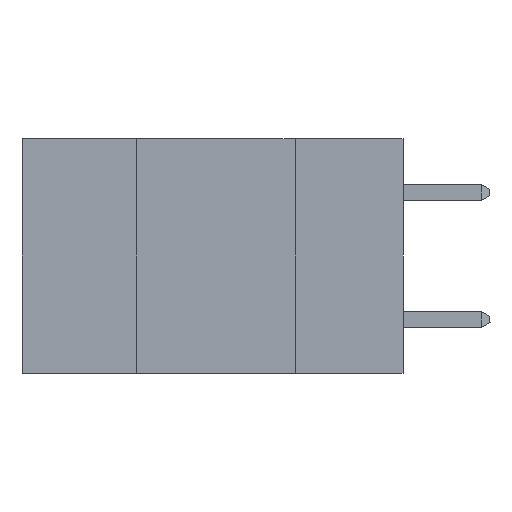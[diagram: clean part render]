
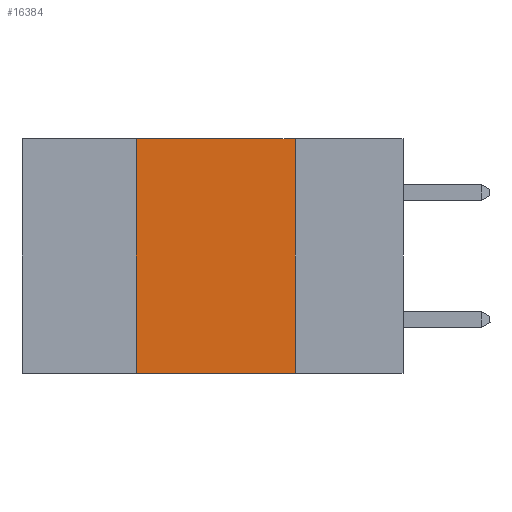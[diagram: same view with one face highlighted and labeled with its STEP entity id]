
A CAD part, left-side view. The second image highlights one B-rep face of the part: STEP entity #16384.
In plain terms, the highlighted planar face has unit normal (-1, 0, 0).
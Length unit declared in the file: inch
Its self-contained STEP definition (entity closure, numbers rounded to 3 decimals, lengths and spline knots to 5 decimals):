
#132 = VECTOR ( 'NONE', #25095, 39.37008 ) ;
#1493 = EDGE_CURVE ( 'NONE', #26820, #26989, #27148, .T. ) ;
#1561 = VECTOR ( 'NONE', #2965, 39.37008 ) ;
#2715 = FACE_OUTER_BOUND ( 'NONE', #10659, .T. ) ;
#2769 = EDGE_CURVE ( 'NONE', #18246, #26820, #4227, .T. ) ;
#2965 = DIRECTION ( 'NONE',  ( 0., -1., 0. ) ) ;
#3888 = CARTESIAN_POINT ( 'NONE',  ( 0., 0.6, 0. ) ) ;
#3927 = CARTESIAN_POINT ( 'NONE',  ( 0., 0.17, -0.37 ) ) ;
#4227 = LINE ( 'NONE', #23454, #10595 ) ;
#6184 = PLANE ( 'NONE',  #26119 ) ;
#7702 = VECTOR ( 'NONE', #22078, 39.37008 ) ;
#9961 = ORIENTED_EDGE ( 'NONE', *, *, #22333, .T. ) ;
#10376 = ORIENTED_EDGE ( 'NONE', *, *, #23019, .F. ) ;
#10595 = VECTOR ( 'NONE', #27329, 39.37008 ) ;
#10659 = EDGE_LOOP ( 'NONE', ( #10376, #29652, #22907, #9961 ) ) ;
#12278 = CARTESIAN_POINT ( 'NONE',  ( 0., 0.6, 0. ) ) ;
#12984 = LINE ( 'NONE', #13124, #132 ) ;
#13124 = CARTESIAN_POINT ( 'NONE',  ( 0., 0.17, 0. ) ) ;
#13564 = DIRECTION ( 'NONE',  ( 0., 0., -1. ) ) ;
#15533 = VERTEX_POINT ( 'NONE', #3927 ) ;
#16384 = ADVANCED_FACE ( 'NONE', ( #2715 ), #6184, .F. ) ;
#18246 = VERTEX_POINT ( 'NONE', #22735 ) ;
#19755 = CARTESIAN_POINT ( 'NONE',  ( 0., 0.6, -0.37 ) ) ;
#22078 = DIRECTION ( 'NONE',  ( 0., -1., 0. ) ) ;
#22333 = EDGE_CURVE ( 'NONE', #18246, #15533, #26512, .T. ) ;
#22735 = CARTESIAN_POINT ( 'NONE',  ( 0., 0.42, -0.37 ) ) ;
#22907 = ORIENTED_EDGE ( 'NONE', *, *, #2769, .F. ) ;
#23019 = EDGE_CURVE ( 'NONE', #26989, #15533, #12984, .T. ) ;
#23123 = DIRECTION ( 'NONE',  ( 1., 0., 0. ) ) ;
#23454 = CARTESIAN_POINT ( 'NONE',  ( 0., 0.42, 0. ) ) ;
#25024 = CARTESIAN_POINT ( 'NONE',  ( 0., 0.42, 0. ) ) ;
#25095 = DIRECTION ( 'NONE',  ( 0., 0., -1. ) ) ;
#26119 = AXIS2_PLACEMENT_3D ( 'NONE', #3888, #23123, #13564 ) ;
#26512 = LINE ( 'NONE', #19755, #7702 ) ;
#26820 = VERTEX_POINT ( 'NONE', #25024 ) ;
#26989 = VERTEX_POINT ( 'NONE', #27766 ) ;
#27148 = LINE ( 'NONE', #12278, #1561 ) ;
#27329 = DIRECTION ( 'NONE',  ( 0., 0., 1. ) ) ;
#27766 = CARTESIAN_POINT ( 'NONE',  ( 0., 0.17, 0. ) ) ;
#29652 = ORIENTED_EDGE ( 'NONE', *, *, #1493, .F. ) ;
